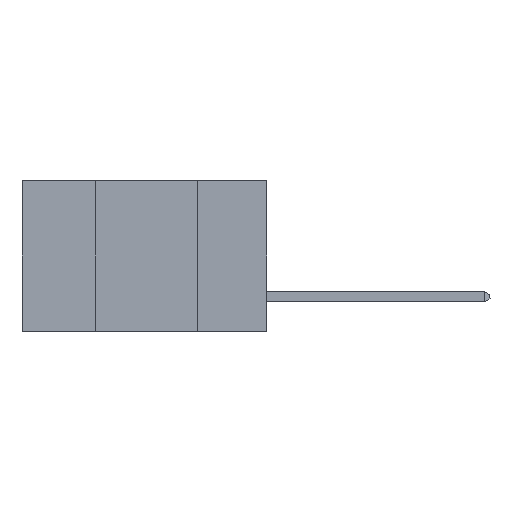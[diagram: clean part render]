
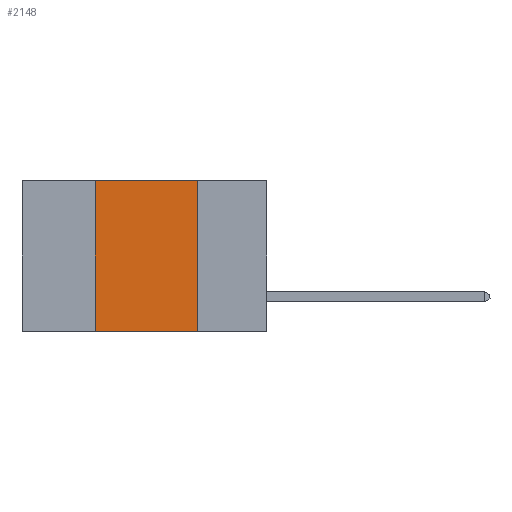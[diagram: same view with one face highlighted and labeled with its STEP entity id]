
A CAD part, left-side view. The second image highlights one B-rep face of the part: STEP entity #2148.
In plain terms, the highlighted planar face has unit normal (-1, 0, 0).
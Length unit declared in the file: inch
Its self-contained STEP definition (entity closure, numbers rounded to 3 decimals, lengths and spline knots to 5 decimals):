
#1006 = CARTESIAN_POINT ( 'NONE',  ( 0., 0.42, 0. ) ) ;
#1324 = CARTESIAN_POINT ( 'NONE',  ( 0., 0.6, 0. ) ) ;
#1359 = VERTEX_POINT ( 'NONE', #1006 ) ;
#1423 = LINE ( 'NONE', #6472, #5675 ) ;
#1547 = DIRECTION ( 'NONE',  ( 0., 0., 1. ) ) ;
#1710 = VERTEX_POINT ( 'NONE', #8747 ) ;
#2148 = ADVANCED_FACE ( 'NONE', ( #5887 ), #10409, .F. ) ;
#2497 = CARTESIAN_POINT ( 'NONE',  ( 0., 0.17, 0. ) ) ;
#2740 = EDGE_CURVE ( 'NONE', #5710, #1710, #4218, .T. ) ;
#3102 = VECTOR ( 'NONE', #6378, 39.37008 ) ;
#3214 = CARTESIAN_POINT ( 'NONE',  ( 0., 0.42, -0.37 ) ) ;
#3706 = AXIS2_PLACEMENT_3D ( 'NONE', #9613, #9778, #6954 ) ;
#4218 = LINE ( 'NONE', #5548, #9940 ) ;
#4234 = ORIENTED_EDGE ( 'NONE', *, *, #5146, .F. ) ;
#4300 = EDGE_CURVE ( 'NONE', #7549, #1710, #1423, .T. ) ;
#5146 = EDGE_CURVE ( 'NONE', #7549, #1359, #10369, .T. ) ;
#5548 = CARTESIAN_POINT ( 'NONE',  ( 0., 0.17, 0. ) ) ;
#5675 = VECTOR ( 'NONE', #9180, 39.37008 ) ;
#5710 = VERTEX_POINT ( 'NONE', #2497 ) ;
#5887 = FACE_OUTER_BOUND ( 'NONE', #10412, .T. ) ;
#6378 = DIRECTION ( 'NONE',  ( 0., -1., 0. ) ) ;
#6472 = CARTESIAN_POINT ( 'NONE',  ( 0., 0.6, -0.37 ) ) ;
#6609 = DIRECTION ( 'NONE',  ( 0., 0., -1. ) ) ;
#6954 = DIRECTION ( 'NONE',  ( 0., 0., -1. ) ) ;
#7197 = ORIENTED_EDGE ( 'NONE', *, *, #8593, .F. ) ;
#7549 = VERTEX_POINT ( 'NONE', #3214 ) ;
#8593 = EDGE_CURVE ( 'NONE', #1359, #5710, #9381, .T. ) ;
#8623 = ORIENTED_EDGE ( 'NONE', *, *, #4300, .T. ) ;
#8747 = CARTESIAN_POINT ( 'NONE',  ( 0., 0.17, -0.37 ) ) ;
#8826 = CARTESIAN_POINT ( 'NONE',  ( 0., 0.42, 0. ) ) ;
#8840 = ORIENTED_EDGE ( 'NONE', *, *, #2740, .F. ) ;
#9180 = DIRECTION ( 'NONE',  ( 0., -1., 0. ) ) ;
#9381 = LINE ( 'NONE', #1324, #3102 ) ;
#9613 = CARTESIAN_POINT ( 'NONE',  ( 0., 0.6, 0. ) ) ;
#9660 = VECTOR ( 'NONE', #1547, 39.37008 ) ;
#9778 = DIRECTION ( 'NONE',  ( 1., 0., 0. ) ) ;
#9940 = VECTOR ( 'NONE', #6609, 39.37008 ) ;
#10369 = LINE ( 'NONE', #8826, #9660 ) ;
#10409 = PLANE ( 'NONE',  #3706 ) ;
#10412 = EDGE_LOOP ( 'NONE', ( #8840, #7197, #4234, #8623 ) ) ;
